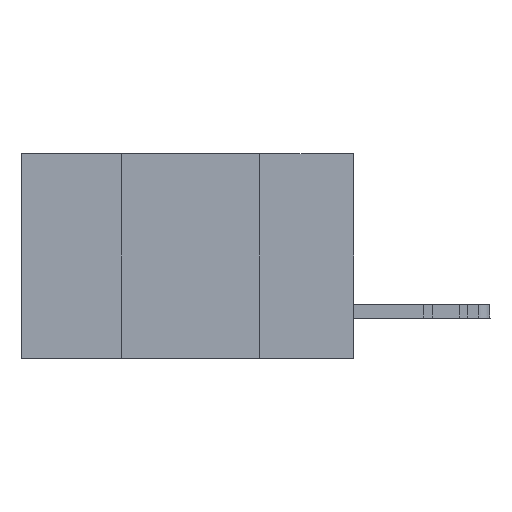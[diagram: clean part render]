
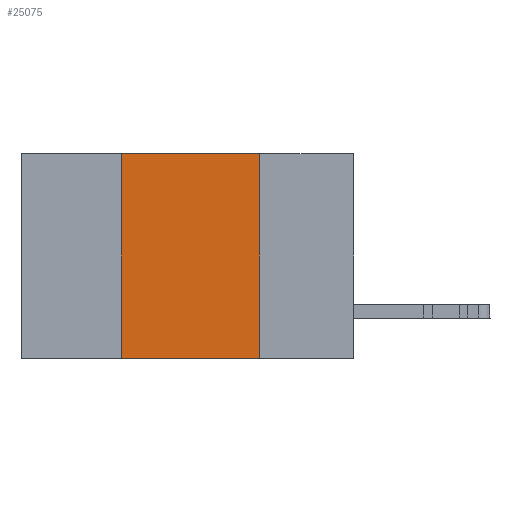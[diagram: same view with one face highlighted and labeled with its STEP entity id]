
A CAD part, left-side view. The second image highlights one B-rep face of the part: STEP entity #25075.
In plain terms, the highlighted planar face has unit normal (-1, 0, 0).
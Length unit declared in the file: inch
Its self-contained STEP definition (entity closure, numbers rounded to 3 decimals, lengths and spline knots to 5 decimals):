
#1127 = ORIENTED_EDGE ( 'NONE', *, *, #23557, .F. ) ;
#1361 = ORIENTED_EDGE ( 'NONE', *, *, #10689, .T. ) ;
#2383 = LINE ( 'NONE', #20688, #46468 ) ;
#5221 = VERTEX_POINT ( 'NONE', #32612 ) ;
#10689 = EDGE_CURVE ( 'NONE', #28764, #28640, #11003, .T. ) ;
#11003 = LINE ( 'NONE', #39694, #14242 ) ;
#11191 = FACE_OUTER_BOUND ( 'NONE', #21600, .T. ) ;
#11668 = DIRECTION ( 'NONE',  ( 1., 0., 0. ) ) ;
#12567 = CARTESIAN_POINT ( 'NONE',  ( 0., 0.42, -0.37 ) ) ;
#13100 = DIRECTION ( 'NONE',  ( 0., 0., 1. ) ) ;
#14242 = VECTOR ( 'NONE', #25467, 39.37008 ) ;
#16117 = AXIS2_PLACEMENT_3D ( 'NONE', #33456, #11668, #40587 ) ;
#16994 = CARTESIAN_POINT ( 'NONE',  ( 0., 0.17, 0. ) ) ;
#17439 = CARTESIAN_POINT ( 'NONE',  ( 0., 0.17, 0. ) ) ;
#17450 = DIRECTION ( 'NONE',  ( 0., 0., -1. ) ) ;
#18010 = VERTEX_POINT ( 'NONE', #17439 ) ;
#18079 = CARTESIAN_POINT ( 'NONE',  ( 0., 0.6, 0. ) ) ;
#20551 = LINE ( 'NONE', #16994, #22778 ) ;
#20688 = CARTESIAN_POINT ( 'NONE',  ( 0., 0.42, 0. ) ) ;
#20954 = DIRECTION ( 'NONE',  ( 0., -1., 0. ) ) ;
#21600 = EDGE_LOOP ( 'NONE', ( #28606, #29183, #1127, #1361 ) ) ;
#22778 = VECTOR ( 'NONE', #17450, 39.37008 ) ;
#23557 = EDGE_CURVE ( 'NONE', #28764, #5221, #2383, .T. ) ;
#24412 = VECTOR ( 'NONE', #20954, 39.37008 ) ;
#25075 = ADVANCED_FACE ( 'NONE', ( #11191 ), #36555, .F. ) ;
#25161 = CARTESIAN_POINT ( 'NONE',  ( 0., 0.17, -0.37 ) ) ;
#25467 = DIRECTION ( 'NONE',  ( 0., -1., 0. ) ) ;
#28606 = ORIENTED_EDGE ( 'NONE', *, *, #43551, .F. ) ;
#28640 = VERTEX_POINT ( 'NONE', #25161 ) ;
#28764 = VERTEX_POINT ( 'NONE', #12567 ) ;
#29183 = ORIENTED_EDGE ( 'NONE', *, *, #32910, .F. ) ;
#32612 = CARTESIAN_POINT ( 'NONE',  ( 0., 0.42, 0. ) ) ;
#32910 = EDGE_CURVE ( 'NONE', #5221, #18010, #43463, .T. ) ;
#33456 = CARTESIAN_POINT ( 'NONE',  ( 0., 0.6, 0. ) ) ;
#36555 = PLANE ( 'NONE',  #16117 ) ;
#39694 = CARTESIAN_POINT ( 'NONE',  ( 0., 0.6, -0.37 ) ) ;
#40587 = DIRECTION ( 'NONE',  ( 0., 0., -1. ) ) ;
#43463 = LINE ( 'NONE', #18079, #24412 ) ;
#43551 = EDGE_CURVE ( 'NONE', #18010, #28640, #20551, .T. ) ;
#46468 = VECTOR ( 'NONE', #13100, 39.37008 ) ;
